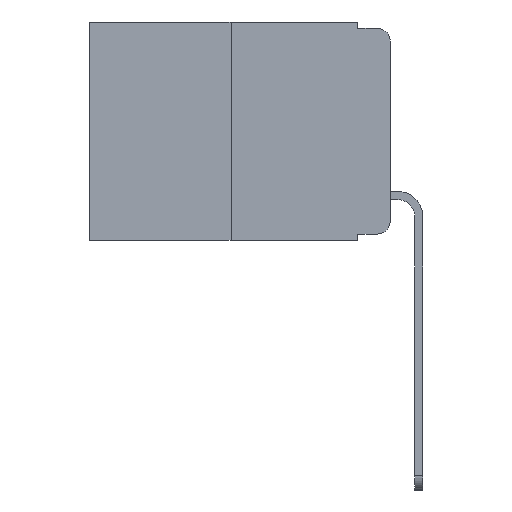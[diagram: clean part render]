
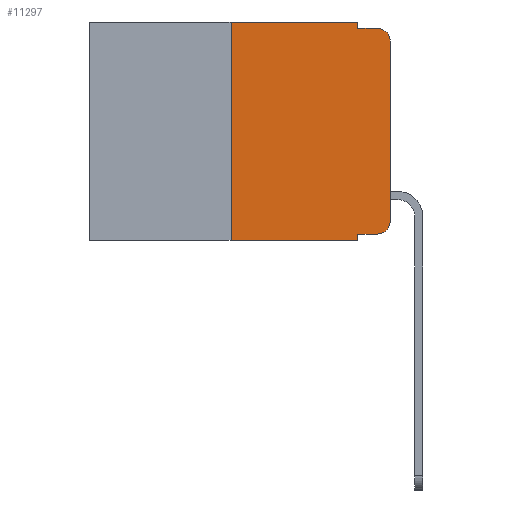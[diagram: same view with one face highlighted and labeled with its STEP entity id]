
A CAD part, left-side view. The second image highlights one B-rep face of the part: STEP entity #11297.
In plain terms, the highlighted planar face has unit normal (-1, 0, 0).
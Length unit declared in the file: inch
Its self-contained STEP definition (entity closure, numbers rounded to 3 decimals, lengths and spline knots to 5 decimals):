
#3 = VERTEX_POINT ( 'NONE', #697 ) ;
#697 = CARTESIAN_POINT ( 'NONE',  ( 0., 0.051, -0.01 ) ) ;
#977 = EDGE_CURVE ( 'NONE', #3422, #13622, #25337, .T. ) ;
#1262 = EDGE_CURVE ( 'NONE', #3, #2735, #8767, .T. ) ;
#1396 = VECTOR ( 'NONE', #10369, 39.37008 ) ;
#1460 = DIRECTION ( 'NONE',  ( 1., 0., 0. ) ) ;
#2735 = VERTEX_POINT ( 'NONE', #19923 ) ;
#2905 = DIRECTION ( 'NONE',  ( 0., 0., -1. ) ) ;
#3422 = VERTEX_POINT ( 'NONE', #7353 ) ;
#3587 = LINE ( 'NONE', #23774, #23549 ) ;
#3749 = CARTESIAN_POINT ( 'NONE',  ( 0., 0.051, -0.01 ) ) ;
#4114 = CARTESIAN_POINT ( 'NONE',  ( 0., 0., -0.313 ) ) ;
#4229 = VECTOR ( 'NONE', #19434, 39.37008 ) ;
#4300 = CARTESIAN_POINT ( 'NONE',  ( 0., 0.25, 0. ) ) ;
#5190 = EDGE_CURVE ( 'NONE', #17248, #14751, #7089, .T. ) ;
#5623 = CARTESIAN_POINT ( 'NONE',  ( 0., 0.051, 0. ) ) ;
#5817 = ORIENTED_EDGE ( 'NONE', *, *, #21626, .T. ) ;
#6460 = FACE_OUTER_BOUND ( 'NONE', #21393, .T. ) ;
#6986 = CARTESIAN_POINT ( 'NONE',  ( 0., 0.051, -0.333 ) ) ;
#7089 = LINE ( 'NONE', #6986, #8616 ) ;
#7353 = CARTESIAN_POINT ( 'NONE',  ( 0., 0.25, -0.343 ) ) ;
#7409 = DIRECTION ( 'NONE',  ( 0., 0., -1. ) ) ;
#7492 = CARTESIAN_POINT ( 'NONE',  ( 0., 0.473, 0. ) ) ;
#7871 = AXIS2_PLACEMENT_3D ( 'NONE', #8351, #16518, #18557 ) ;
#8351 = CARTESIAN_POINT ( 'NONE',  ( 0., 0.02, -0.03 ) ) ;
#8616 = VECTOR ( 'NONE', #19697, 39.37008 ) ;
#8767 = LINE ( 'NONE', #3749, #13463 ) ;
#9394 = CARTESIAN_POINT ( 'NONE',  ( 0., 0.473, -0.343 ) ) ;
#9926 = CARTESIAN_POINT ( 'NONE',  ( 0., 0., 0. ) ) ;
#10369 = DIRECTION ( 'NONE',  ( 0., 0., -1. ) ) ;
#10473 = ORIENTED_EDGE ( 'NONE', *, *, #22947, .F. ) ;
#10524 = VECTOR ( 'NONE', #13504, 39.37008 ) ;
#11297 = ADVANCED_FACE ( 'NONE', ( #6460 ), #24931, .F. ) ;
#11920 = CIRCLE ( 'NONE', #12732, 0.02 ) ;
#12367 = EDGE_CURVE ( 'NONE', #19183, #22705, #13252, .T. ) ;
#12530 = CARTESIAN_POINT ( 'NONE',  ( 0., 0.02, -0.313 ) ) ;
#12732 = AXIS2_PLACEMENT_3D ( 'NONE', #12530, #18559, #2905 ) ;
#13252 = LINE ( 'NONE', #9926, #23226 ) ;
#13356 = ORIENTED_EDGE ( 'NONE', *, *, #19577, .F. ) ;
#13463 = VECTOR ( 'NONE', #17708, 39.37008 ) ;
#13504 = DIRECTION ( 'NONE',  ( 0., -1., 0. ) ) ;
#13622 = VERTEX_POINT ( 'NONE', #16462 ) ;
#13782 = ORIENTED_EDGE ( 'NONE', *, *, #5190, .T. ) ;
#14596 = ORIENTED_EDGE ( 'NONE', *, *, #15735, .T. ) ;
#14751 = VERTEX_POINT ( 'NONE', #21633 ) ;
#14894 = ORIENTED_EDGE ( 'NONE', *, *, #12367, .T. ) ;
#14925 = ORIENTED_EDGE ( 'NONE', *, *, #1262, .F. ) ;
#14959 = ORIENTED_EDGE ( 'NONE', *, *, #23460, .F. ) ;
#15735 = EDGE_CURVE ( 'NONE', #14751, #19183, #11920, .T. ) ;
#16258 = VECTOR ( 'NONE', #22346, 39.37008 ) ;
#16418 = VERTEX_POINT ( 'NONE', #5623 ) ;
#16462 = CARTESIAN_POINT ( 'NONE',  ( 0., 0.25, 0. ) ) ;
#16518 = DIRECTION ( 'NONE',  ( -1., 0., 0. ) ) ;
#16637 = ORIENTED_EDGE ( 'NONE', *, *, #21306, .T. ) ;
#16684 = LINE ( 'NONE', #18227, #1396 ) ;
#17248 = VERTEX_POINT ( 'NONE', #18383 ) ;
#17649 = LINE ( 'NONE', #19701, #4229 ) ;
#17708 = DIRECTION ( 'NONE',  ( 0., -1., 0. ) ) ;
#17948 = DIRECTION ( 'NONE',  ( 0., 0., 1. ) ) ;
#18028 = DIRECTION ( 'NONE',  ( 0., -1., 0. ) ) ;
#18227 = CARTESIAN_POINT ( 'NONE',  ( 0., 0.051, 0. ) ) ;
#18295 = CARTESIAN_POINT ( 'NONE',  ( 0., 0.051, -0.343 ) ) ;
#18352 = AXIS2_PLACEMENT_3D ( 'NONE', #7492, #1460, #7409 ) ;
#18383 = CARTESIAN_POINT ( 'NONE',  ( 0., 0.051, -0.333 ) ) ;
#18557 = DIRECTION ( 'NONE',  ( 0., 0., -1. ) ) ;
#18559 = DIRECTION ( 'NONE',  ( -1., 0., 0. ) ) ;
#19162 = ORIENTED_EDGE ( 'NONE', *, *, #977, .F. ) ;
#19183 = VERTEX_POINT ( 'NONE', #4114 ) ;
#19434 = DIRECTION ( 'NONE',  ( 0., 0., -1. ) ) ;
#19577 = EDGE_CURVE ( 'NONE', #17248, #21574, #17649, .T. ) ;
#19697 = DIRECTION ( 'NONE',  ( 0., -1., 0. ) ) ;
#19701 = CARTESIAN_POINT ( 'NONE',  ( 0., 0.051, 0. ) ) ;
#19923 = CARTESIAN_POINT ( 'NONE',  ( 0., 0.02, -0.01 ) ) ;
#21306 = EDGE_CURVE ( 'NONE', #3422, #21574, #24552, .T. ) ;
#21393 = EDGE_LOOP ( 'NONE', ( #14894, #5817, #14925, #10473, #14959, #19162, #16637, #13356, #13782, #14596 ) ) ;
#21574 = VERTEX_POINT ( 'NONE', #18295 ) ;
#21626 = EDGE_CURVE ( 'NONE', #22705, #2735, #22041, .T. ) ;
#21633 = CARTESIAN_POINT ( 'NONE',  ( 0., 0.02, -0.333 ) ) ;
#22041 = CIRCLE ( 'NONE', #7871, 0.02 ) ;
#22346 = DIRECTION ( 'NONE',  ( 0., 0., 1. ) ) ;
#22705 = VERTEX_POINT ( 'NONE', #23988 ) ;
#22947 = EDGE_CURVE ( 'NONE', #16418, #3, #16684, .T. ) ;
#23226 = VECTOR ( 'NONE', #17948, 39.37008 ) ;
#23460 = EDGE_CURVE ( 'NONE', #13622, #16418, #3587, .T. ) ;
#23549 = VECTOR ( 'NONE', #18028, 39.37008 ) ;
#23774 = CARTESIAN_POINT ( 'NONE',  ( 0., 0.473, 0. ) ) ;
#23988 = CARTESIAN_POINT ( 'NONE',  ( 0., 0., -0.03 ) ) ;
#24552 = LINE ( 'NONE', #9394, #10524 ) ;
#24931 = PLANE ( 'NONE',  #18352 ) ;
#25337 = LINE ( 'NONE', #4300, #16258 ) ;
